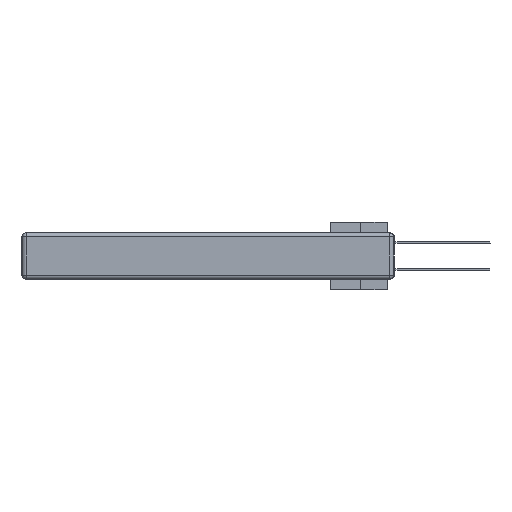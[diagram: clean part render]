
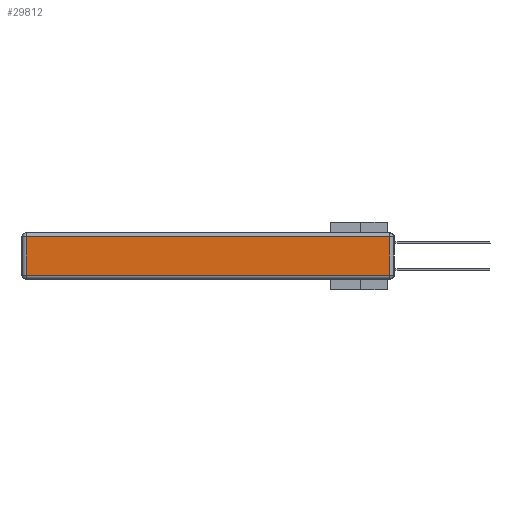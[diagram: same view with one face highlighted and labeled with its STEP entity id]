
A CAD part, left-side view. The second image highlights one B-rep face of the part: STEP entity #29812.
In plain terms, the highlighted planar face has unit normal (-1, 0, 0).
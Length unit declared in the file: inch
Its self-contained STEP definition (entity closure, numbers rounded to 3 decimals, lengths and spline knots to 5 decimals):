
#463 = EDGE_CURVE ( 'NONE', #6368, #3979, #712, .T. ) ;
#712 = LINE ( 'NONE', #10506, #29770 ) ;
#1419 = CARTESIAN_POINT ( 'NONE',  ( 0., 0., -0.343 ) ) ;
#2100 = ORIENTED_EDGE ( 'NONE', *, *, #6414, .T. ) ;
#2230 = VECTOR ( 'NONE', #19994, 39.37008 ) ;
#2568 = CARTESIAN_POINT ( 'NONE',  ( 0., 2.72, -0.313 ) ) ;
#3046 = ORIENTED_EDGE ( 'NONE', *, *, #4299, .T. ) ;
#3204 = LINE ( 'NONE', #25872, #2230 ) ;
#3979 = VERTEX_POINT ( 'NONE', #14010 ) ;
#4135 = EDGE_CURVE ( 'NONE', #26157, #6368, #22167, .T. ) ;
#4299 = EDGE_CURVE ( 'NONE', #22614, #26157, #20072, .T. ) ;
#5518 = CARTESIAN_POINT ( 'NONE',  ( 0., 2.72, -0.343 ) ) ;
#6368 = VERTEX_POINT ( 'NONE', #31409 ) ;
#6414 = EDGE_CURVE ( 'NONE', #3979, #22614, #3204, .T. ) ;
#10506 = CARTESIAN_POINT ( 'NONE',  ( 0., 0.03, -0.343 ) ) ;
#13040 = DIRECTION ( 'NONE',  ( 0., 0., -1. ) ) ;
#14010 = CARTESIAN_POINT ( 'NONE',  ( 0., 0.03, -0.03 ) ) ;
#14467 = EDGE_LOOP ( 'NONE', ( #27643, #15263, #2100, #3046 ) ) ;
#15263 = ORIENTED_EDGE ( 'NONE', *, *, #463, .T. ) ;
#15517 = PLANE ( 'NONE',  #28540 ) ;
#15988 = DIRECTION ( 'NONE',  ( -1., 0., 0. ) ) ;
#17338 = CARTESIAN_POINT ( 'NONE',  ( 0., 0., -0.313 ) ) ;
#18058 = DIRECTION ( 'NONE',  ( 0., 0., 1. ) ) ;
#19157 = VECTOR ( 'NONE', #13040, 39.37008 ) ;
#19994 = DIRECTION ( 'NONE',  ( 0., 1., 0. ) ) ;
#20072 = LINE ( 'NONE', #5518, #19157 ) ;
#21690 = DIRECTION ( 'NONE',  ( 0., -1., 0. ) ) ;
#22167 = LINE ( 'NONE', #17338, #23786 ) ;
#22614 = VERTEX_POINT ( 'NONE', #26637 ) ;
#23028 = FACE_OUTER_BOUND ( 'NONE', #14467, .T. ) ;
#23786 = VECTOR ( 'NONE', #21690, 39.37008 ) ;
#25872 = CARTESIAN_POINT ( 'NONE',  ( 0., 2.75, -0.03 ) ) ;
#26157 = VERTEX_POINT ( 'NONE', #2568 ) ;
#26637 = CARTESIAN_POINT ( 'NONE',  ( 0., 2.72, -0.03 ) ) ;
#27643 = ORIENTED_EDGE ( 'NONE', *, *, #4135, .T. ) ;
#28540 = AXIS2_PLACEMENT_3D ( 'NONE', #1419, #15988, #18058 ) ;
#29770 = VECTOR ( 'NONE', #30042, 39.37008 ) ;
#29812 = ADVANCED_FACE ( 'NONE', ( #23028 ), #15517, .T. ) ;
#30042 = DIRECTION ( 'NONE',  ( 0., 0., 1. ) ) ;
#31409 = CARTESIAN_POINT ( 'NONE',  ( 0., 0.03, -0.313 ) ) ;
